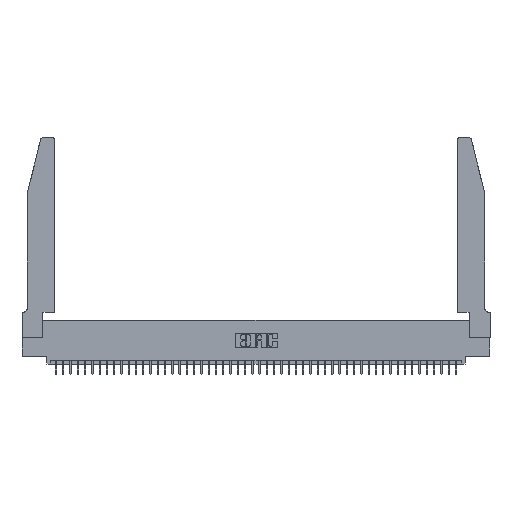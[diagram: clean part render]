
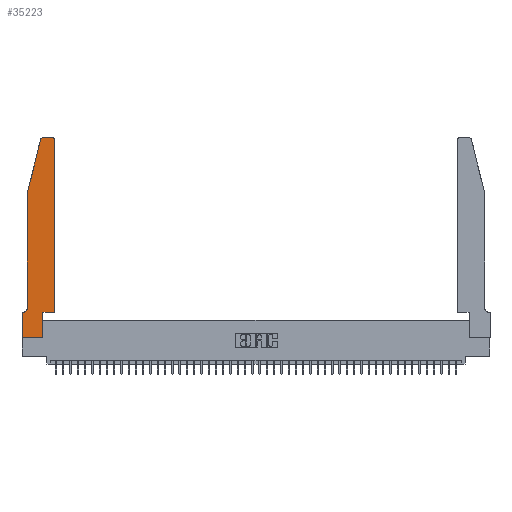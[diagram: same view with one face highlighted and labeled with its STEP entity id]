
A CAD part, top view. The second image highlights one B-rep face of the part: STEP entity #35223.
In plain terms, the highlighted planar face has unit normal (0, 0, 1).
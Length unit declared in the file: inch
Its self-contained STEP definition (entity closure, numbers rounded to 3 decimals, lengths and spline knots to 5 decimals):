
#219 = LINE ( 'NONE', #43343, #21421 ) ;
#257 = CARTESIAN_POINT ( 'NONE',  ( 0.284, 2.72, 0.37 ) ) ;
#554 = VERTEX_POINT ( 'NONE', #44925 ) ;
#682 = VERTEX_POINT ( 'NONE', #39165 ) ;
#762 = CIRCLE ( 'NONE', #43308, 0.03 ) ;
#1969 = CARTESIAN_POINT ( 'NONE',  ( 0., 0.35, 0.37 ) ) ;
#2702 = CARTESIAN_POINT ( 'NONE',  ( 0.4205, 2.72, 0.37 ) ) ;
#2777 = EDGE_CURVE ( 'NONE', #29456, #38637, #9103, .T. ) ;
#3033 = VECTOR ( 'NONE', #29663, 39.37008 ) ;
#3287 = ORIENTED_EDGE ( 'NONE', *, *, #12970, .T. ) ;
#3577 = DIRECTION ( 'NONE',  ( 1., 0., 0. ) ) ;
#4693 = DIRECTION ( 'NONE',  ( 0., 1., 0. ) ) ;
#4919 = AXIS2_PLACEMENT_3D ( 'NONE', #2702, #6061, #20332 ) ;
#5235 = AXIS2_PLACEMENT_3D ( 'NONE', #45536, #12674, #5293 ) ;
#5237 = CARTESIAN_POINT ( 'NONE',  ( 0.4505, 0.35, 0.37 ) ) ;
#5293 = DIRECTION ( 'NONE',  ( -1., 0., 0. ) ) ;
#5833 = VERTEX_POINT ( 'NONE', #18853 ) ;
#6061 = DIRECTION ( 'NONE',  ( 0., 0., 1. ) ) ;
#6524 = ORIENTED_EDGE ( 'NONE', *, *, #27163, .T. ) ;
#6916 = CARTESIAN_POINT ( 'NONE',  ( 0., 0., 0.37 ) ) ;
#6942 = CARTESIAN_POINT ( 'NONE',  ( 0.0755, 0.42, 0.37 ) ) ;
#7646 = CARTESIAN_POINT ( 'NONE',  ( 0.4205, 2.75, 0.37 ) ) ;
#9103 = LINE ( 'NONE', #34812, #28983 ) ;
#10251 = CIRCLE ( 'NONE', #4919, 0.03 ) ;
#10377 = ORIENTED_EDGE ( 'NONE', *, *, #14013, .T. ) ;
#11141 = VERTEX_POINT ( 'NONE', #5237 ) ;
#11701 = LINE ( 'NONE', #15049, #24230 ) ;
#12674 = DIRECTION ( 'NONE',  ( 0., 0., -1. ) ) ;
#12970 = EDGE_CURVE ( 'NONE', #25167, #5833, #11701, .T. ) ;
#13149 = DIRECTION ( 'NONE',  ( -1., 0., 0. ) ) ;
#13945 = DIRECTION ( 'NONE',  ( -1., 0., 0. ) ) ;
#14013 = EDGE_CURVE ( 'NONE', #22317, #682, #41098, .T. ) ;
#14337 = CIRCLE ( 'NONE', #5235, 0.07 ) ;
#14352 = EDGE_CURVE ( 'NONE', #38637, #25167, #762, .T. ) ;
#14642 = CARTESIAN_POINT ( 'NONE',  ( 0.0055, 0.35, 0.37 ) ) ;
#15049 = CARTESIAN_POINT ( 'NONE',  ( 0.0755, 2., 0.37 ) ) ;
#15289 = DIRECTION ( 'NONE',  ( 0., 0., 1. ) ) ;
#15845 = VERTEX_POINT ( 'NONE', #14642 ) ;
#16266 = CARTESIAN_POINT ( 'NONE',  ( 0.284, 2.75, 0.37 ) ) ;
#17313 = EDGE_CURVE ( 'NONE', #46173, #22317, #219, .T. ) ;
#17847 = DIRECTION ( 'NONE',  ( 0., -1., 0. ) ) ;
#18684 = CARTESIAN_POINT ( 'NONE',  ( 0.2865, 0., 0.37 ) ) ;
#18853 = CARTESIAN_POINT ( 'NONE',  ( 0.0755, 2., 0.37 ) ) ;
#20332 = DIRECTION ( 'NONE',  ( 1., 0., 0. ) ) ;
#21421 = VECTOR ( 'NONE', #3577, 39.37008 ) ;
#22317 = VERTEX_POINT ( 'NONE', #18684 ) ;
#22372 = DIRECTION ( 'NONE',  ( -0.239, -0.971, 0. ) ) ;
#22374 = VERTEX_POINT ( 'NONE', #42810 ) ;
#22642 = EDGE_CURVE ( 'NONE', #22374, #29456, #10251, .T. ) ;
#22751 = LINE ( 'NONE', #37311, #40333 ) ;
#23839 = DIRECTION ( 'NONE',  ( 0., 0., 1. ) ) ;
#24207 = ORIENTED_EDGE ( 'NONE', *, *, #40823, .T. ) ;
#24230 = VECTOR ( 'NONE', #22372, 39.37008 ) ;
#25167 = VERTEX_POINT ( 'NONE', #37011 ) ;
#25211 = LINE ( 'NONE', #6916, #32591 ) ;
#25621 = LINE ( 'NONE', #36118, #37070 ) ;
#25900 = ORIENTED_EDGE ( 'NONE', *, *, #27354, .T. ) ;
#25913 = EDGE_CURVE ( 'NONE', #682, #11141, #25621, .T. ) ;
#26086 = CARTESIAN_POINT ( 'NONE',  ( 0.2865, 0.35, 0.37 ) ) ;
#26176 = AXIS2_PLACEMENT_3D ( 'NONE', #1969, #23839, #28120 ) ;
#26249 = ORIENTED_EDGE ( 'NONE', *, *, #22642, .T. ) ;
#26419 = ORIENTED_EDGE ( 'NONE', *, *, #17313, .T. ) ;
#27163 = EDGE_CURVE ( 'NONE', #45619, #15845, #14337, .T. ) ;
#27286 = ORIENTED_EDGE ( 'NONE', *, *, #43781, .T. ) ;
#27354 = EDGE_CURVE ( 'NONE', #554, #46173, #25211, .T. ) ;
#27491 = CARTESIAN_POINT ( 'NONE',  ( 0.0755, 0.35, 0.37 ) ) ;
#28120 = DIRECTION ( 'NONE',  ( 1., 0., 0. ) ) ;
#28983 = VECTOR ( 'NONE', #13149, 39.37008 ) ;
#29456 = VERTEX_POINT ( 'NONE', #7646 ) ;
#29663 = DIRECTION ( 'NONE',  ( 0., 1., 0. ) ) ;
#30193 = VECTOR ( 'NONE', #13945, 39.37008 ) ;
#32591 = VECTOR ( 'NONE', #17847, 39.37008 ) ;
#33987 = CARTESIAN_POINT ( 'NONE',  ( 0.0755, 2., 0.37 ) ) ;
#34143 = CARTESIAN_POINT ( 'NONE',  ( 0., 0., 0.37 ) ) ;
#34812 = CARTESIAN_POINT ( 'NONE',  ( 0.2605, 2.75, 0.37 ) ) ;
#35223 = ADVANCED_FACE ( 'NONE', ( #46253 ), #42666, .T. ) ;
#36118 = CARTESIAN_POINT ( 'NONE',  ( 0.4505, 0.35, 0.37 ) ) ;
#36129 = ORIENTED_EDGE ( 'NONE', *, *, #43714, .T. ) ;
#36580 = EDGE_LOOP ( 'NONE', ( #37624, #37828, #3287, #36129, #6524, #24207, #25900, #26419, #10377, #45002, #27286, #26249 ) ) ;
#36705 = DIRECTION ( 'NONE',  ( 1., 0., 0. ) ) ;
#37011 = CARTESIAN_POINT ( 'NONE',  ( 0.25487, 2.72718, 0.37 ) ) ;
#37070 = VECTOR ( 'NONE', #40163, 39.37008 ) ;
#37311 = CARTESIAN_POINT ( 'NONE',  ( 0.4505, 0.35, 0.37 ) ) ;
#37624 = ORIENTED_EDGE ( 'NONE', *, *, #2777, .T. ) ;
#37828 = ORIENTED_EDGE ( 'NONE', *, *, #14352, .T. ) ;
#38637 = VERTEX_POINT ( 'NONE', #16266 ) ;
#39165 = CARTESIAN_POINT ( 'NONE',  ( 0.2865, 0.35, 0.37 ) ) ;
#40163 = DIRECTION ( 'NONE',  ( 1., 0., 0. ) ) ;
#40333 = VECTOR ( 'NONE', #4693, 39.37008 ) ;
#40823 = EDGE_CURVE ( 'NONE', #15845, #554, #46551, .T. ) ;
#41098 = LINE ( 'NONE', #26086, #3033 ) ;
#41333 = DIRECTION ( 'NONE',  ( 0., -1., 0. ) ) ;
#42666 = PLANE ( 'NONE',  #26176 ) ;
#42810 = CARTESIAN_POINT ( 'NONE',  ( 0.4505, 2.72, 0.37 ) ) ;
#43308 = AXIS2_PLACEMENT_3D ( 'NONE', #257, #15289, #36705 ) ;
#43343 = CARTESIAN_POINT ( 'NONE',  ( 0., 0., 0.37 ) ) ;
#43714 = EDGE_CURVE ( 'NONE', #5833, #45619, #44696, .T. ) ;
#43781 = EDGE_CURVE ( 'NONE', #11141, #22374, #22751, .T. ) ;
#44696 = LINE ( 'NONE', #33987, #46386 ) ;
#44925 = CARTESIAN_POINT ( 'NONE',  ( 0., 0.35, 0.37 ) ) ;
#45002 = ORIENTED_EDGE ( 'NONE', *, *, #25913, .T. ) ;
#45536 = CARTESIAN_POINT ( 'NONE',  ( 0.0055, 0.42, 0.37 ) ) ;
#45619 = VERTEX_POINT ( 'NONE', #6942 ) ;
#46173 = VERTEX_POINT ( 'NONE', #34143 ) ;
#46253 = FACE_OUTER_BOUND ( 'NONE', #36580, .T. ) ;
#46386 = VECTOR ( 'NONE', #41333, 39.37008 ) ;
#46551 = LINE ( 'NONE', #27491, #30193 ) ;
